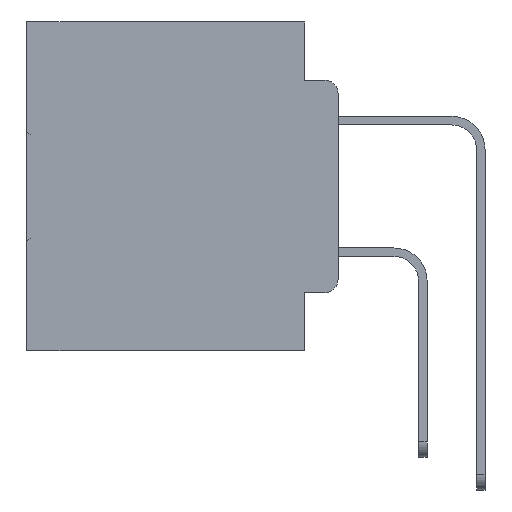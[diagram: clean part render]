
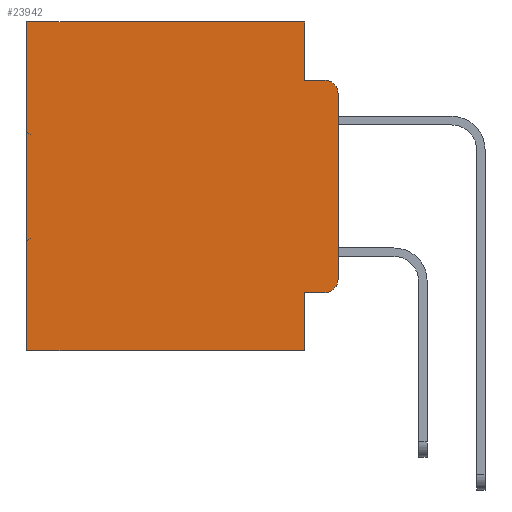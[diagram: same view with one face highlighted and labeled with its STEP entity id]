
A CAD part, left-side view. The second image highlights one B-rep face of the part: STEP entity #23942.
In plain terms, the highlighted planar face has unit normal (-1, 0, 0).
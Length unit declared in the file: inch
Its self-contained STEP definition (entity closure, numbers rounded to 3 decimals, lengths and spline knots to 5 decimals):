
#14 = EDGE_CURVE ( 'NONE', #36408, #6015, #35065, .T. ) ;
#18 = ORIENTED_EDGE ( 'NONE', *, *, #30740, .F. ) ;
#503 = CARTESIAN_POINT ( 'NONE',  ( 0.298, 0., 0. ) ) ;
#1584 = CARTESIAN_POINT ( 'NONE',  ( 0.298, 0., 0. ) ) ;
#2660 = CARTESIAN_POINT ( 'NONE',  ( 0.298, 0.02, -0.1085 ) ) ;
#2709 = VECTOR ( 'NONE', #32787, 39.37008 ) ;
#3318 = VECTOR ( 'NONE', #11197, 39.37008 ) ;
#3438 = ORIENTED_EDGE ( 'NONE', *, *, #12225, .F. ) ;
#4033 = CARTESIAN_POINT ( 'NONE',  ( 0.298, 0., 0. ) ) ;
#4444 = ORIENTED_EDGE ( 'NONE', *, *, #25567, .F. ) ;
#4507 = AXIS2_PLACEMENT_3D ( 'NONE', #29873, #12887, #32697 ) ;
#5466 = LINE ( 'NONE', #503, #20568 ) ;
#5548 = DIRECTION ( 'NONE',  ( 0., 0., -1. ) ) ;
#6015 = VERTEX_POINT ( 'NONE', #10368 ) ;
#6676 = ORIENTED_EDGE ( 'NONE', *, *, #29347, .T. ) ;
#7204 = ORIENTED_EDGE ( 'NONE', *, *, #14, .T. ) ;
#7213 = VERTEX_POINT ( 'NONE', #24570 ) ;
#7500 = DIRECTION ( 'NONE',  ( 0., -1., 0. ) ) ;
#8402 = CARTESIAN_POINT ( 'NONE',  ( 0.298, 0., -0.5 ) ) ;
#8708 = VERTEX_POINT ( 'NONE', #30238 ) ;
#9605 = LINE ( 'NONE', #18313, #10472 ) ;
#9730 = DIRECTION ( 'NONE',  ( 0., 0., -1. ) ) ;
#9791 = VECTOR ( 'NONE', #35706, 39.37008 ) ;
#10339 = EDGE_CURVE ( 'NONE', #23765, #22071, #5466, .T. ) ;
#10368 = CARTESIAN_POINT ( 'NONE',  ( 0.298, 0.473, 0. ) ) ;
#10472 = VECTOR ( 'NONE', #9730, 39.37008 ) ;
#10654 = LINE ( 'NONE', #32940, #9791 ) ;
#11197 = DIRECTION ( 'NONE',  ( 0., 1., 0. ) ) ;
#11619 = VECTOR ( 'NONE', #7500, 39.37008 ) ;
#11824 = ORIENTED_EDGE ( 'NONE', *, *, #16006, .T. ) ;
#12225 = EDGE_CURVE ( 'NONE', #7213, #26059, #10654, .T. ) ;
#12529 = DIRECTION ( 'NONE',  ( 1., 0., 0. ) ) ;
#12887 = DIRECTION ( 'NONE',  ( -1., 0., 0. ) ) ;
#13202 = FACE_OUTER_BOUND ( 'NONE', #14815, .T. ) ;
#13416 = CARTESIAN_POINT ( 'NONE',  ( 0.298, 0.473, -0.5 ) ) ;
#13499 = VECTOR ( 'NONE', #17285, 39.37008 ) ;
#14815 = EDGE_LOOP ( 'NONE', ( #24753, #11824, #3438, #30191, #7204, #26668, #18, #4444, #27082, #6676 ) ) ;
#15956 = AXIS2_PLACEMENT_3D ( 'NONE', #4033, #12529, #32334 ) ;
#16006 = EDGE_CURVE ( 'NONE', #23765, #26059, #21024, .T. ) ;
#16916 = CARTESIAN_POINT ( 'NONE',  ( 0.298, 0.02, -0.4115 ) ) ;
#16946 = CARTESIAN_POINT ( 'NONE',  ( 0.298, 0., -0.3915 ) ) ;
#17285 = DIRECTION ( 'NONE',  ( 0., 0., -1. ) ) ;
#17817 = LINE ( 'NONE', #27145, #2709 ) ;
#18313 = CARTESIAN_POINT ( 'NONE',  ( 0.298, 0.473, 0. ) ) ;
#19120 = DIRECTION ( 'NONE',  ( 0., 1., 0. ) ) ;
#19217 = LINE ( 'NONE', #32939, #11619 ) ;
#19904 = EDGE_CURVE ( 'NONE', #6015, #30624, #9605, .T. ) ;
#20149 = VECTOR ( 'NONE', #19120, 39.37008 ) ;
#20299 = CARTESIAN_POINT ( 'NONE',  ( 0.298, 0., -0.1085 ) ) ;
#20408 = DIRECTION ( 'NONE',  ( 0., 0., -1. ) ) ;
#20568 = VECTOR ( 'NONE', #20408, 39.37008 ) ;
#21024 = CIRCLE ( 'NONE', #34461, 0.02 ) ;
#21801 = EDGE_CURVE ( 'NONE', #36408, #7213, #17817, .T. ) ;
#22043 = LINE ( 'NONE', #25733, #13499 ) ;
#22071 = VERTEX_POINT ( 'NONE', #16946 ) ;
#22551 = DIRECTION ( 'NONE',  ( -1., 0., 0. ) ) ;
#23765 = VERTEX_POINT ( 'NONE', #20299 ) ;
#23844 = PLANE ( 'NONE',  #15956 ) ;
#23942 = ADVANCED_FACE ( 'NONE', ( #13202 ), #23844, .F. ) ;
#24570 = CARTESIAN_POINT ( 'NONE',  ( 0.298, 0.051, -0.0885 ) ) ;
#24753 = ORIENTED_EDGE ( 'NONE', *, *, #10339, .F. ) ;
#24757 = CARTESIAN_POINT ( 'NONE',  ( 0.298, 0.051, -0.5 ) ) ;
#25156 = CARTESIAN_POINT ( 'NONE',  ( 0.298, 0.051, 0. ) ) ;
#25567 = EDGE_CURVE ( 'NONE', #8708, #26885, #22043, .T. ) ;
#25733 = CARTESIAN_POINT ( 'NONE',  ( 0.298, 0.051, 0. ) ) ;
#25944 = LINE ( 'NONE', #8402, #3318 ) ;
#26059 = VERTEX_POINT ( 'NONE', #26411 ) ;
#26411 = CARTESIAN_POINT ( 'NONE',  ( 0.298, 0.02, -0.0885 ) ) ;
#26668 = ORIENTED_EDGE ( 'NONE', *, *, #19904, .T. ) ;
#26885 = VERTEX_POINT ( 'NONE', #24757 ) ;
#27082 = ORIENTED_EDGE ( 'NONE', *, *, #27435, .T. ) ;
#27145 = CARTESIAN_POINT ( 'NONE',  ( 0.298, 0.051, 0. ) ) ;
#27435 = EDGE_CURVE ( 'NONE', #8708, #31952, #19217, .T. ) ;
#29347 = EDGE_CURVE ( 'NONE', #31952, #22071, #33500, .T. ) ;
#29873 = CARTESIAN_POINT ( 'NONE',  ( 0.298, 0.02, -0.3915 ) ) ;
#30191 = ORIENTED_EDGE ( 'NONE', *, *, #21801, .F. ) ;
#30238 = CARTESIAN_POINT ( 'NONE',  ( 0.298, 0.051, -0.4115 ) ) ;
#30624 = VERTEX_POINT ( 'NONE', #13416 ) ;
#30740 = EDGE_CURVE ( 'NONE', #26885, #30624, #25944, .T. ) ;
#31952 = VERTEX_POINT ( 'NONE', #16916 ) ;
#32334 = DIRECTION ( 'NONE',  ( 0., 0., -1. ) ) ;
#32697 = DIRECTION ( 'NONE',  ( 0., 0., -1. ) ) ;
#32787 = DIRECTION ( 'NONE',  ( 0., 0., -1. ) ) ;
#32939 = CARTESIAN_POINT ( 'NONE',  ( 0.298, 0.051, -0.4115 ) ) ;
#32940 = CARTESIAN_POINT ( 'NONE',  ( 0.298, 0.051, -0.0885 ) ) ;
#33500 = CIRCLE ( 'NONE', #4507, 0.02 ) ;
#34461 = AXIS2_PLACEMENT_3D ( 'NONE', #2660, #22551, #5548 ) ;
#35065 = LINE ( 'NONE', #1584, #20149 ) ;
#35706 = DIRECTION ( 'NONE',  ( 0., -1., 0. ) ) ;
#36408 = VERTEX_POINT ( 'NONE', #25156 ) ;
